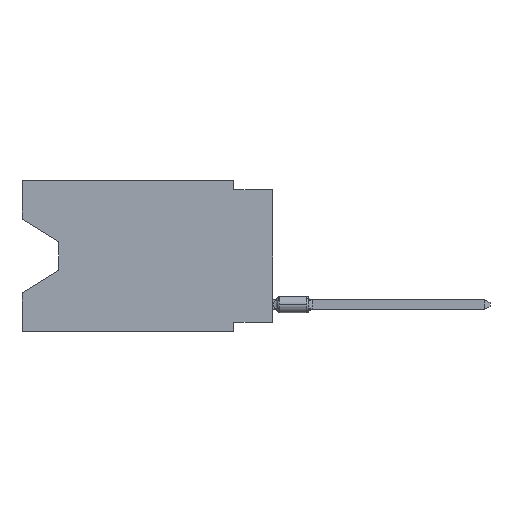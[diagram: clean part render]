
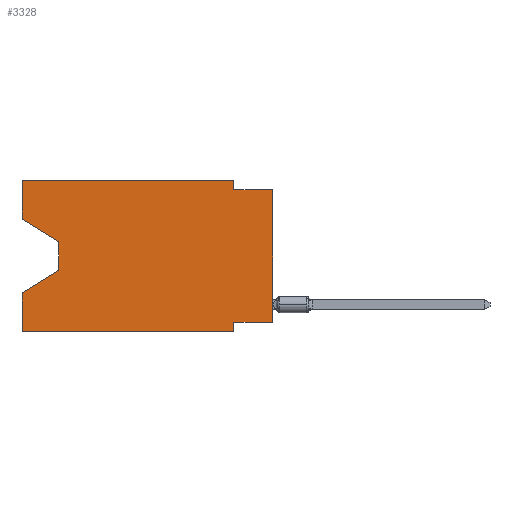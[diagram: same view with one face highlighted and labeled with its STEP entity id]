
A CAD part, left-side view. The second image highlights one B-rep face of the part: STEP entity #3328.
In plain terms, the highlighted planar face has unit normal (-1, 0, 0).
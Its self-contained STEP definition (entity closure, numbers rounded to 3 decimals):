
#26 = EDGE_CURVE ( 'NONE', #17659, #11397, #14218, .T. ) ;
#35 = DIRECTION ( 'NONE',  ( 1., 0., 0. ) ) ;
#44 = ORIENTED_EDGE ( 'NONE', *, *, #6705, .F. ) ;
#92 = VERTEX_POINT ( 'NONE', #12451 ) ;
#224 = FACE_OUTER_BOUND ( 'NONE', #18489, .T. ) ;
#532 = VECTOR ( 'NONE', #8531, 1000. ) ;
#664 = DIRECTION ( 'NONE',  ( 0., 0., -1. ) ) ;
#816 = VECTOR ( 'NONE', #9265, 1000. ) ;
#1280 = VERTEX_POINT ( 'NONE', #16932 ) ;
#1461 = CARTESIAN_POINT ( 'NONE',  ( 0., 16.383, -9.906 ) ) ;
#1618 = PLANE ( 'NONE',  #6511 ) ;
#1617 = CARTESIAN_POINT ( 'NONE',  ( 0., 16.383, -2.546 ) ) ;
#2008 = CARTESIAN_POINT ( 'NONE',  ( 0., 16.383, 0. ) ) ;
#2320 = LINE ( 'NONE', #9766, #7401 ) ;
#2417 = DIRECTION ( 'NONE',  ( 0., -1., 0. ) ) ;
#2775 = CARTESIAN_POINT ( 'NONE',  ( 0., 2.54, 0. ) ) ;
#3328 = ADVANCED_FACE ( 'NONE', ( #224 ), #1618, .F. ) ;
#3529 = LINE ( 'NONE', #14188, #4337 ) ;
#3537 = ORIENTED_EDGE ( 'NONE', *, *, #11301, .F. ) ;
#3699 = EDGE_CURVE ( 'NONE', #15389, #6655, #8359, .T. ) ;
#3773 = DIRECTION ( 'NONE',  ( 0., 0., 1. ) ) ;
#4058 = LINE ( 'NONE', #2775, #12618 ) ;
#4337 = VECTOR ( 'NONE', #664, 1000. ) ;
#4437 = CARTESIAN_POINT ( 'NONE',  ( 0., 2.54, -9.271 ) ) ;
#4478 = CARTESIAN_POINT ( 'NONE',  ( 0., 16.383, 0. ) ) ;
#4504 = LINE ( 'NONE', #15345, #12847 ) ;
#4706 = CARTESIAN_POINT ( 'NONE',  ( 0., 13.97, -4.013 ) ) ;
#5113 = DIRECTION ( 'NONE',  ( 0., 0., -1. ) ) ;
#5327 = ORIENTED_EDGE ( 'NONE', *, *, #6207, .T. ) ;
#5399 = VECTOR ( 'NONE', #5113, 1000. ) ;
#5762 = CARTESIAN_POINT ( 'NONE',  ( 0., 13.97, -5.893 ) ) ;
#5833 = VECTOR ( 'NONE', #10543, 1000. ) ;
#5901 = DIRECTION ( 'NONE',  ( 0., 0., 1. ) ) ;
#5973 = LINE ( 'NONE', #4478, #5833 ) ;
#6207 = EDGE_CURVE ( 'NONE', #14424, #12395, #10661, .T. ) ;
#6255 = DIRECTION ( 'NONE',  ( 0., -0.855, -0.519 ) ) ;
#6360 = CARTESIAN_POINT ( 'NONE',  ( 0., 0., -9.271 ) ) ;
#6511 = AXIS2_PLACEMENT_3D ( 'NONE', #15524, #35, #9252 ) ;
#6655 = VERTEX_POINT ( 'NONE', #11030 ) ;
#6705 = EDGE_CURVE ( 'NONE', #6655, #6955, #9441, .T. ) ;
#6909 = ORIENTED_EDGE ( 'NONE', *, *, #14466, .T. ) ;
#6955 = VERTEX_POINT ( 'NONE', #7611 ) ;
#7082 = ORIENTED_EDGE ( 'NONE', *, *, #18652, .F. ) ;
#7218 = VERTEX_POINT ( 'NONE', #4437 ) ;
#7259 = CARTESIAN_POINT ( 'NONE',  ( 0., 0., -9.271 ) ) ;
#7401 = VECTOR ( 'NONE', #2417, 1000. ) ;
#7611 = CARTESIAN_POINT ( 'NONE',  ( 0., 2.54, 0. ) ) ;
#8208 = EDGE_CURVE ( 'NONE', #9869, #1280, #4504, .T. ) ;
#8359 = LINE ( 'NONE', #17407, #17629 ) ;
#8531 = DIRECTION ( 'NONE',  ( 0., 0.855, -0.519 ) ) ;
#8974 = LINE ( 'NONE', #6360, #15274 ) ;
#9252 = DIRECTION ( 'NONE',  ( 0., 0., -1. ) ) ;
#9265 = DIRECTION ( 'NONE',  ( 0., -1., 0. ) ) ;
#9326 = VECTOR ( 'NONE', #6255, 1000. ) ;
#9378 = CARTESIAN_POINT ( 'NONE',  ( 0., 2.54, -9.906 ) ) ;
#9441 = LINE ( 'NONE', #2008, #19209 ) ;
#9563 = ORIENTED_EDGE ( 'NONE', *, *, #8208, .T. ) ;
#9766 = CARTESIAN_POINT ( 'NONE',  ( 0., 0., -0.635 ) ) ;
#9869 = VERTEX_POINT ( 'NONE', #7259 ) ;
#10174 = EDGE_CURVE ( 'NONE', #6955, #15774, #4058, .T. ) ;
#10543 = DIRECTION ( 'NONE',  ( 0., 0., 1. ) ) ;
#10661 = LINE ( 'NONE', #16740, #816 ) ;
#11030 = CARTESIAN_POINT ( 'NONE',  ( 0., 16.383, 0. ) ) ;
#11301 = EDGE_CURVE ( 'NONE', #7218, #12395, #3529, .T. ) ;
#11397 = VERTEX_POINT ( 'NONE', #12114 ) ;
#12114 = CARTESIAN_POINT ( 'NONE',  ( 0., 16.383, -7.36 ) ) ;
#12166 = ORIENTED_EDGE ( 'NONE', *, *, #10174, .F. ) ;
#12186 = ORIENTED_EDGE ( 'NONE', *, *, #17058, .T. ) ;
#12395 = VERTEX_POINT ( 'NONE', #9378 ) ;
#12451 = CARTESIAN_POINT ( 'NONE',  ( 0., 13.97, -4.013 ) ) ;
#12469 = LINE ( 'NONE', #4706, #5399 ) ;
#12618 = VECTOR ( 'NONE', #13405, 1000. ) ;
#12847 = VECTOR ( 'NONE', #5901, 1000. ) ;
#13405 = DIRECTION ( 'NONE',  ( 0., 0., -1. ) ) ;
#13847 = DIRECTION ( 'NONE',  ( 0., 1., 0. ) ) ;
#14188 = CARTESIAN_POINT ( 'NONE',  ( 0., 2.54, -9.906 ) ) ;
#14218 = LINE ( 'NONE', #17083, #532 ) ;
#14424 = VERTEX_POINT ( 'NONE', #1461 ) ;
#14466 = EDGE_CURVE ( 'NONE', #92, #17659, #12469, .T. ) ;
#15274 = VECTOR ( 'NONE', #13847, 1000. ) ;
#15345 = CARTESIAN_POINT ( 'NONE',  ( 0., 0., 0. ) ) ;
#15389 = VERTEX_POINT ( 'NONE', #17707 ) ;
#15510 = DIRECTION ( 'NONE',  ( 0., -1., 0. ) ) ;
#15524 = CARTESIAN_POINT ( 'NONE',  ( 0., 16.383, 0. ) ) ;
#15774 = VERTEX_POINT ( 'NONE', #19475 ) ;
#16315 = EDGE_CURVE ( 'NONE', #15774, #1280, #2320, .T. ) ;
#16740 = CARTESIAN_POINT ( 'NONE',  ( 0., 16.383, -9.906 ) ) ;
#16932 = CARTESIAN_POINT ( 'NONE',  ( 0., 0., -0.635 ) ) ;
#17058 = EDGE_CURVE ( 'NONE', #15389, #92, #18116, .T. ) ;
#17083 = CARTESIAN_POINT ( 'NONE',  ( 0., 13.97, -5.893 ) ) ;
#17099 = EDGE_CURVE ( 'NONE', #14424, #11397, #5973, .T. ) ;
#17407 = CARTESIAN_POINT ( 'NONE',  ( 0., 16.383, 0. ) ) ;
#17629 = VECTOR ( 'NONE', #3773, 1000. ) ;
#17659 = VERTEX_POINT ( 'NONE', #5762 ) ;
#17707 = CARTESIAN_POINT ( 'NONE',  ( 0., 16.383, -2.546 ) ) ;
#17765 = ORIENTED_EDGE ( 'NONE', *, *, #16315, .F. ) ;
#18116 = LINE ( 'NONE', #1617, #9326 ) ;
#18489 = EDGE_LOOP ( 'NONE', ( #12186, #6909, #19025, #18517, #5327, #3537, #7082, #9563, #17765, #12166, #44, #18922 ) ) ;
#18517 = ORIENTED_EDGE ( 'NONE', *, *, #17099, .F. ) ;
#18652 = EDGE_CURVE ( 'NONE', #9869, #7218, #8974, .T. ) ;
#18922 = ORIENTED_EDGE ( 'NONE', *, *, #3699, .F. ) ;
#19025 = ORIENTED_EDGE ( 'NONE', *, *, #26, .T. ) ;
#19209 = VECTOR ( 'NONE', #15510, 1000. ) ;
#19475 = CARTESIAN_POINT ( 'NONE',  ( 0., 2.54, -0.635 ) ) ;
